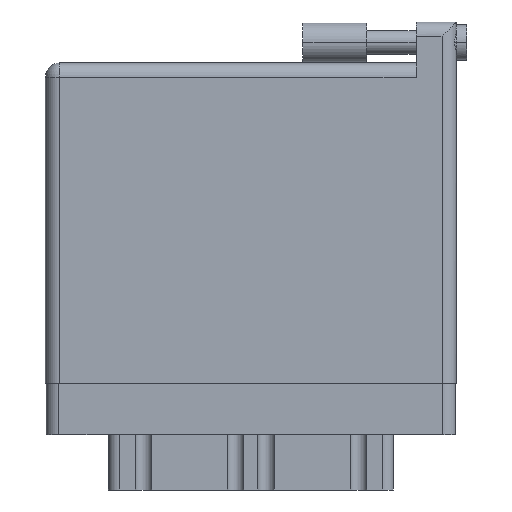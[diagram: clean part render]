
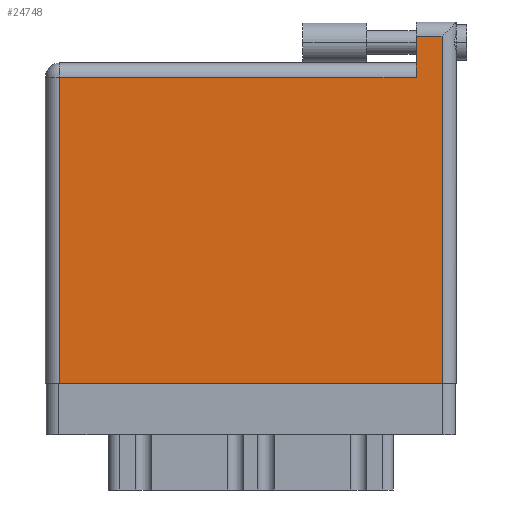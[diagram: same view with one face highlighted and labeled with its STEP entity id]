
A CAD part, front view. The second image highlights one B-rep face of the part: STEP entity #24748.
In plain terms, the highlighted face is planar.
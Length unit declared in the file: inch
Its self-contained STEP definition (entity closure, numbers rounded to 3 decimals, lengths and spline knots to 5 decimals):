
#967 = ORIENTED_EDGE ( 'NONE', *, *, #5009, .T. ) ;
#1089 = EDGE_LOOP ( 'NONE', ( #32526, #1890, #32811, #25240, #967, #14801 ) ) ;
#1688 = CARTESIAN_POINT ( 'NONE',  ( 0.07, 0., 0. ) ) ;
#1890 = ORIENTED_EDGE ( 'NONE', *, *, #21566, .T. ) ;
#2031 = CARTESIAN_POINT ( 'NONE',  ( 1.938, 0., 0. ) ) ;
#3966 = LINE ( 'NONE', #9549, #25683 ) ;
#4545 = VECTOR ( 'NONE', #25403, 39.37008 ) ;
#5009 = EDGE_CURVE ( 'NONE', #25422, #14404, #25205, .T. ) ;
#5043 = EDGE_CURVE ( 'NONE', #14404, #30361, #30252, .T. ) ;
#5062 = DIRECTION ( 'NONE',  ( 0., 1., 0. ) ) ;
#5086 = PLANE ( 'NONE',  #14018 ) ;
#5427 = FACE_OUTER_BOUND ( 'NONE', #1089, .T. ) ;
#5437 = CARTESIAN_POINT ( 'NONE',  ( 0.07, 0., 0. ) ) ;
#6412 = CARTESIAN_POINT ( 'NONE',  ( 1.811, 1.766, 0. ) ) ;
#9549 = CARTESIAN_POINT ( 'NONE',  ( 0., 0., 0. ) ) ;
#10492 = DIRECTION ( 'NONE',  ( -1., 0., 0. ) ) ;
#11378 = EDGE_CURVE ( 'NONE', #15351, #17432, #21373, .T. ) ;
#12812 = CARTESIAN_POINT ( 'NONE',  ( 1.811, 1.496, 0. ) ) ;
#13280 = CARTESIAN_POINT ( 'NONE',  ( 0., 1.566, 0. ) ) ;
#13773 = LINE ( 'NONE', #18321, #30839 ) ;
#13839 = CARTESIAN_POINT ( 'NONE',  ( 1.938, 1.696, 0. ) ) ;
#14018 = AXIS2_PLACEMENT_3D ( 'NONE', #13280, #24072, #10492 ) ;
#14404 = VERTEX_POINT ( 'NONE', #27147 ) ;
#14604 = DIRECTION ( 'NONE',  ( 1., 0., 0. ) ) ;
#14801 = ORIENTED_EDGE ( 'NONE', *, *, #5043, .T. ) ;
#15351 = VERTEX_POINT ( 'NONE', #13839 ) ;
#15721 = VERTEX_POINT ( 'NONE', #2031 ) ;
#16715 = LINE ( 'NONE', #6412, #4545 ) ;
#17432 = VERTEX_POINT ( 'NONE', #32668 ) ;
#18321 = CARTESIAN_POINT ( 'NONE',  ( 1.938, 1.766, 0. ) ) ;
#19645 = DIRECTION ( 'NONE',  ( 0., -1., 0. ) ) ;
#19990 = CARTESIAN_POINT ( 'NONE',  ( 0., 1.496, 0. ) ) ;
#21373 = LINE ( 'NONE', #26416, #31517 ) ;
#21566 = EDGE_CURVE ( 'NONE', #15721, #15351, #13773, .T. ) ;
#24072 = DIRECTION ( 'NONE',  ( 0., 0., -1. ) ) ;
#24748 = ADVANCED_FACE ( 'NONE', ( #5427 ), #5086, .F. ) ;
#25205 = LINE ( 'NONE', #19990, #33868 ) ;
#25240 = ORIENTED_EDGE ( 'NONE', *, *, #27958, .T. ) ;
#25403 = DIRECTION ( 'NONE',  ( 0., -1., 0. ) ) ;
#25422 = VERTEX_POINT ( 'NONE', #12812 ) ;
#25683 = VECTOR ( 'NONE', #14604, 39.37008 ) ;
#26416 = CARTESIAN_POINT ( 'NONE',  ( 0., 1.696, 0. ) ) ;
#27147 = CARTESIAN_POINT ( 'NONE',  ( 0.07, 1.496, 0. ) ) ;
#27198 = VECTOR ( 'NONE', #19645, 39.37008 ) ;
#27807 = DIRECTION ( 'NONE',  ( -1., 0., 0. ) ) ;
#27958 = EDGE_CURVE ( 'NONE', #17432, #25422, #16715, .T. ) ;
#29367 = DIRECTION ( 'NONE',  ( -1., 0., 0. ) ) ;
#30252 = LINE ( 'NONE', #1688, #27198 ) ;
#30361 = VERTEX_POINT ( 'NONE', #5437 ) ;
#30839 = VECTOR ( 'NONE', #5062, 39.37008 ) ;
#31517 = VECTOR ( 'NONE', #29367, 39.37008 ) ;
#32526 = ORIENTED_EDGE ( 'NONE', *, *, #34329, .T. ) ;
#32668 = CARTESIAN_POINT ( 'NONE',  ( 1.811, 1.696, 0. ) ) ;
#32811 = ORIENTED_EDGE ( 'NONE', *, *, #11378, .T. ) ;
#33868 = VECTOR ( 'NONE', #27807, 39.37008 ) ;
#34329 = EDGE_CURVE ( 'NONE', #30361, #15721, #3966, .T. ) ;
